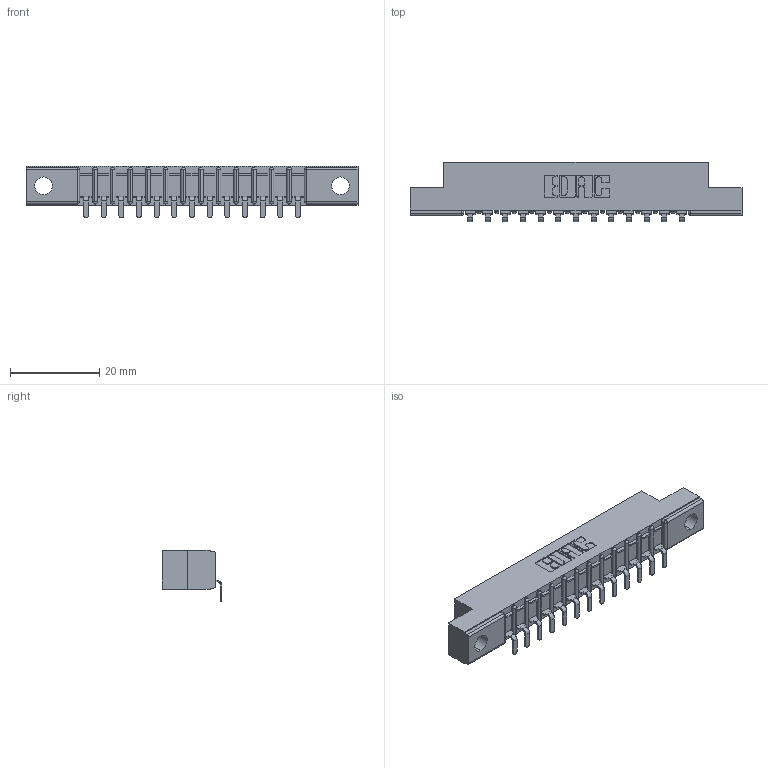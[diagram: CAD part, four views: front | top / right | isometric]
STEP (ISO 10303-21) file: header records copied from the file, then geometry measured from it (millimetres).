
FILE_DESCRIPTION (( 'STEP AP203' ), '1' );
FILE_NAME ('307-013-553-104.STEP', '2019-09-04T20:15:57', ( '' ), ( '' ), 'SwSTEP 2.0', 'SolidWorks 2016', '' );
FILE_SCHEMA (( 'CONFIG_CONTROL_DESIGN' ));
Length unit declared in the file: inch
Products named in the file (3): 307 Part_.156 Dia Mounting Holes; 307-013-553-104; 307-290-002_553
Assembly tree (14 placements, depth 2):
  307-013-553-104
    307 Part_.156 Dia Mounting Holes
    307-290-002_553  x13
Bounding box: 74.52 x 13.32 x 11.51 mm (x, y, z)
Volume: 4809.2 mm3; surface area: 8141.4 mm2
Topology: 14 solids, 14 shells, 1160 faces, 3531 edges, 2314 vertices
Faces by surface type: plane 695, cylinder 437, sphere 28
Entity records: 15992 total; most frequent: CARTESIAN_POINT 2698, ORIENTED_EDGE 2686, DIRECTION 2627, EDGE_CURVE 1343, LINE 1021, VECTOR 1021, VERTEX_POINT 874, AXIS2_PLACEMENT_3D 803
